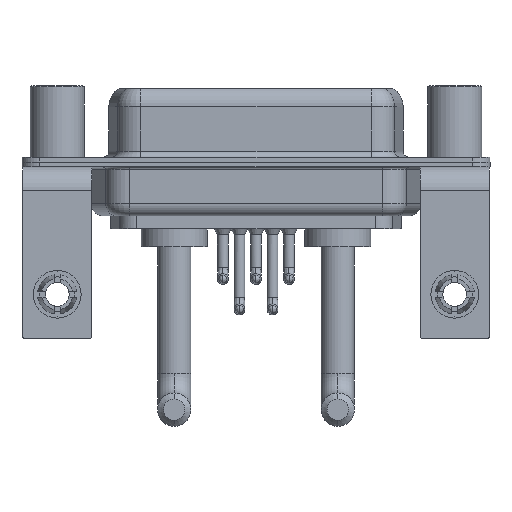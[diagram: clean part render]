
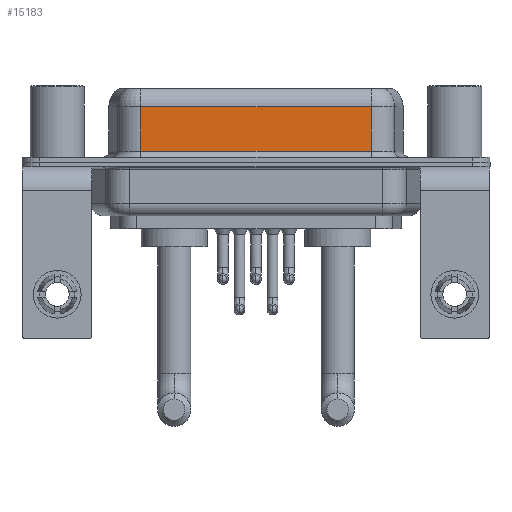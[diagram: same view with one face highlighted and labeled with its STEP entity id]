
A CAD part, front view. The second image highlights one B-rep face of the part: STEP entity #15183.
In plain terms, the highlighted planar face has unit normal (0, -1, 0).
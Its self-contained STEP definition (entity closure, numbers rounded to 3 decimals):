
#185 = VECTOR ( 'NONE', #2340, 1000. ) ;
#533 = VERTEX_POINT ( 'NONE', #9957 ) ;
#1126 = CARTESIAN_POINT ( 'NONE',  ( 26.287, -3.95, 4.65 ) ) ;
#1216 = EDGE_CURVE ( 'NONE', #16197, #14009, #5058, .T. ) ;
#2340 = DIRECTION ( 'NONE',  ( 0., 0., -1. ) ) ;
#2360 = DIRECTION ( 'NONE',  ( 0., 0., -1. ) ) ;
#2447 = LINE ( 'NONE', #3933, #185 ) ;
#3896 = DIRECTION ( 'NONE',  ( -1., 0., 0. ) ) ;
#3933 = CARTESIAN_POINT ( 'NONE',  ( 26.287, -3.95, 6.4 ) ) ;
#4164 = PLANE ( 'NONE',  #18498 ) ;
#4472 = DIRECTION ( 'NONE',  ( 0., 1., 0. ) ) ;
#5058 = LINE ( 'NONE', #11569, #19884 ) ;
#5630 = ORIENTED_EDGE ( 'NONE', *, *, #20988, .F. ) ;
#5645 = CARTESIAN_POINT ( 'NONE',  ( 7.013, -3.95, 6.4 ) ) ;
#6694 = EDGE_CURVE ( 'NONE', #15606, #533, #12204, .T. ) ;
#8424 = CARTESIAN_POINT ( 'NONE',  ( 7.013, -3.95, 0.9 ) ) ;
#9957 = CARTESIAN_POINT ( 'NONE',  ( 7.013, -3.95, 4.65 ) ) ;
#9968 = DIRECTION ( 'NONE',  ( 1., 0., 0. ) ) ;
#10959 = EDGE_CURVE ( 'NONE', #533, #16197, #16908, .T. ) ;
#11569 = CARTESIAN_POINT ( 'NONE',  ( 26.287, -3.95, 0.9 ) ) ;
#11995 = CARTESIAN_POINT ( 'NONE',  ( 26.287, -3.95, 4.65 ) ) ;
#12204 = LINE ( 'NONE', #11995, #15864 ) ;
#12568 = FACE_OUTER_BOUND ( 'NONE', #20987, .T. ) ;
#12581 = ORIENTED_EDGE ( 'NONE', *, *, #10959, .T. ) ;
#14009 = VERTEX_POINT ( 'NONE', #18472 ) ;
#14052 = CARTESIAN_POINT ( 'NONE',  ( 26.287, -3.95, 6.4 ) ) ;
#14644 = VECTOR ( 'NONE', #2360, 1000. ) ;
#15141 = ORIENTED_EDGE ( 'NONE', *, *, #6694, .T. ) ;
#15183 = ADVANCED_FACE ( 'NONE', ( #12568 ), #4164, .F. ) ;
#15606 = VERTEX_POINT ( 'NONE', #1126 ) ;
#15864 = VECTOR ( 'NONE', #3896, 1000. ) ;
#16197 = VERTEX_POINT ( 'NONE', #8424 ) ;
#16581 = ORIENTED_EDGE ( 'NONE', *, *, #1216, .T. ) ;
#16908 = LINE ( 'NONE', #5645, #14644 ) ;
#17450 = DIRECTION ( 'NONE',  ( 0., 0., 1. ) ) ;
#18472 = CARTESIAN_POINT ( 'NONE',  ( 26.287, -3.95, 0.9 ) ) ;
#18498 = AXIS2_PLACEMENT_3D ( 'NONE', #14052, #4472, #17450 ) ;
#19884 = VECTOR ( 'NONE', #9968, 1000. ) ;
#20987 = EDGE_LOOP ( 'NONE', ( #5630, #15141, #12581, #16581 ) ) ;
#20988 = EDGE_CURVE ( 'NONE', #15606, #14009, #2447, .T. ) ;
